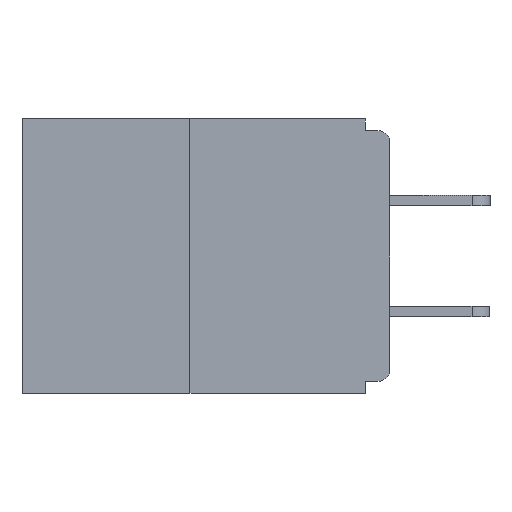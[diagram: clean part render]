
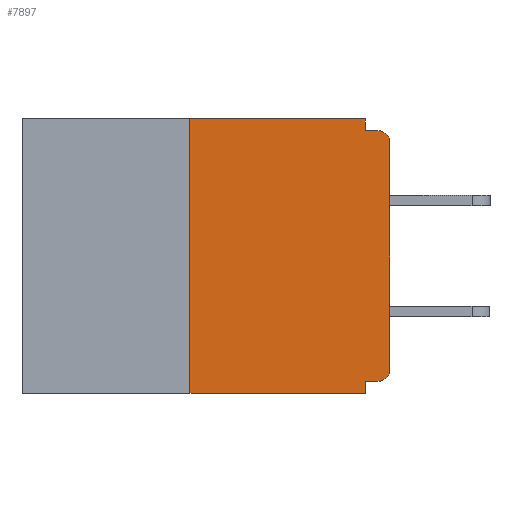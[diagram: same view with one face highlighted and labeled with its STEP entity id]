
A CAD part, left-side view. The second image highlights one B-rep face of the part: STEP entity #7897.
In plain terms, the highlighted planar face has unit normal (-1, 0, 0).
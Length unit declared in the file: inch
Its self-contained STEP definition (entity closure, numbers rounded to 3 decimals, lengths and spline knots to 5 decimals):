
#961 = AXIS2_PLACEMENT_3D ( 'NONE', #22468, #20516, #13202 ) ;
#1058 = CARTESIAN_POINT ( 'NONE',  ( 0., 0.015, -0.313 ) ) ;
#1637 = DIRECTION ( 'NONE',  ( 0., 0., -1. ) ) ;
#2032 = DIRECTION ( 'NONE',  ( 0., 0., 1. ) ) ;
#2103 = CARTESIAN_POINT ( 'NONE',  ( 0., 0.46, 0. ) ) ;
#2160 = VECTOR ( 'NONE', #12771, 39.37008 ) ;
#2252 = CARTESIAN_POINT ( 'NONE',  ( 0., 0.031, -0.015 ) ) ;
#2762 = CARTESIAN_POINT ( 'NONE',  ( 0., 0., -0.328 ) ) ;
#2796 = VERTEX_POINT ( 'NONE', #6605 ) ;
#4033 = CARTESIAN_POINT ( 'NONE',  ( 0., 0., -0.313 ) ) ;
#4126 = LINE ( 'NONE', #11154, #8659 ) ;
#4278 = VECTOR ( 'NONE', #19106, 39.37008 ) ;
#4566 = CARTESIAN_POINT ( 'NONE',  ( 0., 0.015, -0.328 ) ) ;
#4717 = CARTESIAN_POINT ( 'NONE',  ( 0., 0.46, 0. ) ) ;
#4772 = CARTESIAN_POINT ( 'NONE',  ( 0., 0.031, -0.328 ) ) ;
#4995 = LINE ( 'NONE', #21578, #2160 ) ;
#5096 = CARTESIAN_POINT ( 'NONE',  ( 0., 0.031, -0.343 ) ) ;
#5404 = LINE ( 'NONE', #2762, #10468 ) ;
#5552 = CARTESIAN_POINT ( 'NONE',  ( 0., 0.25, 0. ) ) ;
#5697 = DIRECTION ( 'NONE',  ( 0., 0., -1. ) ) ;
#5854 = PLANE ( 'NONE',  #20369 ) ;
#5968 = LINE ( 'NONE', #4717, #4278 ) ;
#6163 = DIRECTION ( 'NONE',  ( 0., 0., -1. ) ) ;
#6268 = CIRCLE ( 'NONE', #8490, 0.015 ) ;
#6605 = CARTESIAN_POINT ( 'NONE',  ( 0., 0.25, 0. ) ) ;
#6688 = ORIENTED_EDGE ( 'NONE', *, *, #12822, .F. ) ;
#6816 = VERTEX_POINT ( 'NONE', #20747 ) ;
#7607 = VECTOR ( 'NONE', #19515, 39.37008 ) ;
#7686 = EDGE_CURVE ( 'NONE', #12947, #17990, #20958, .T. ) ;
#7765 = VECTOR ( 'NONE', #9118, 39.37008 ) ;
#7801 = VERTEX_POINT ( 'NONE', #2252 ) ;
#7897 = ADVANCED_FACE ( 'NONE', ( #8918 ), #5854, .F. ) ;
#7995 = LINE ( 'NONE', #5096, #11646 ) ;
#8466 = ORIENTED_EDGE ( 'NONE', *, *, #16003, .T. ) ;
#8490 = AXIS2_PLACEMENT_3D ( 'NONE', #1058, #17100, #6163 ) ;
#8659 = VECTOR ( 'NONE', #18235, 39.37008 ) ;
#8673 = VECTOR ( 'NONE', #2032, 39.37008 ) ;
#8918 = FACE_OUTER_BOUND ( 'NONE', #12753, .T. ) ;
#8960 = CARTESIAN_POINT ( 'NONE',  ( 0., 0.46, -0.343 ) ) ;
#9011 = EDGE_CURVE ( 'NONE', #11687, #12338, #15322, .T. ) ;
#9102 = VERTEX_POINT ( 'NONE', #4566 ) ;
#9118 = DIRECTION ( 'NONE',  ( 0., -1., 0. ) ) ;
#9491 = LINE ( 'NONE', #5552, #8673 ) ;
#9560 = LINE ( 'NONE', #19280, #7607 ) ;
#9911 = CARTESIAN_POINT ( 'NONE',  ( 0., 0.031, -0.343 ) ) ;
#9999 = DIRECTION ( 'NONE',  ( 0., 1., 0. ) ) ;
#10468 = VECTOR ( 'NONE', #9999, 39.37008 ) ;
#11154 = CARTESIAN_POINT ( 'NONE',  ( 0., 0., 0. ) ) ;
#11646 = VECTOR ( 'NONE', #1637, 39.37008 ) ;
#11687 = VERTEX_POINT ( 'NONE', #15221 ) ;
#12338 = VERTEX_POINT ( 'NONE', #18419 ) ;
#12550 = VERTEX_POINT ( 'NONE', #4772 ) ;
#12753 = EDGE_LOOP ( 'NONE', ( #18655, #6688, #15230, #17712, #17539, #8466, #20015, #14508, #19276, #15536 ) ) ;
#12771 = DIRECTION ( 'NONE',  ( 0., 0., -1. ) ) ;
#12822 = EDGE_CURVE ( 'NONE', #12947, #2796, #9491, .T. ) ;
#12947 = VERTEX_POINT ( 'NONE', #20391 ) ;
#13202 = DIRECTION ( 'NONE',  ( 0., 0., -1. ) ) ;
#14508 = ORIENTED_EDGE ( 'NONE', *, *, #9011, .T. ) ;
#14705 = DIRECTION ( 'NONE',  ( 1., 0., 0. ) ) ;
#15221 = CARTESIAN_POINT ( 'NONE',  ( 0., 0., -0.03 ) ) ;
#15230 = ORIENTED_EDGE ( 'NONE', *, *, #7686, .T. ) ;
#15322 = CIRCLE ( 'NONE', #961, 0.015 ) ;
#15536 = ORIENTED_EDGE ( 'NONE', *, *, #17515, .F. ) ;
#16003 = EDGE_CURVE ( 'NONE', #9102, #20928, #6268, .T. ) ;
#16598 = EDGE_CURVE ( 'NONE', #9102, #12550, #5404, .T. ) ;
#16624 = EDGE_CURVE ( 'NONE', #2796, #6816, #5968, .T. ) ;
#17100 = DIRECTION ( 'NONE',  ( -1., 0., 0. ) ) ;
#17515 = EDGE_CURVE ( 'NONE', #6816, #7801, #4995, .T. ) ;
#17539 = ORIENTED_EDGE ( 'NONE', *, *, #16598, .F. ) ;
#17712 = ORIENTED_EDGE ( 'NONE', *, *, #19796, .F. ) ;
#17990 = VERTEX_POINT ( 'NONE', #9911 ) ;
#18195 = EDGE_CURVE ( 'NONE', #20928, #11687, #4126, .T. ) ;
#18235 = DIRECTION ( 'NONE',  ( 0., 0., 1. ) ) ;
#18419 = CARTESIAN_POINT ( 'NONE',  ( 0., 0.015, -0.015 ) ) ;
#18655 = ORIENTED_EDGE ( 'NONE', *, *, #16624, .F. ) ;
#19106 = DIRECTION ( 'NONE',  ( 0., -1., 0. ) ) ;
#19276 = ORIENTED_EDGE ( 'NONE', *, *, #22598, .F. ) ;
#19280 = CARTESIAN_POINT ( 'NONE',  ( 0., 0., -0.015 ) ) ;
#19515 = DIRECTION ( 'NONE',  ( 0., -1., 0. ) ) ;
#19796 = EDGE_CURVE ( 'NONE', #12550, #17990, #7995, .T. ) ;
#20015 = ORIENTED_EDGE ( 'NONE', *, *, #18195, .T. ) ;
#20369 = AXIS2_PLACEMENT_3D ( 'NONE', #2103, #14705, #5697 ) ;
#20391 = CARTESIAN_POINT ( 'NONE',  ( 0., 0.25, -0.343 ) ) ;
#20516 = DIRECTION ( 'NONE',  ( -1., 0., 0. ) ) ;
#20747 = CARTESIAN_POINT ( 'NONE',  ( 0., 0.031, 0. ) ) ;
#20928 = VERTEX_POINT ( 'NONE', #4033 ) ;
#20958 = LINE ( 'NONE', #8960, #7765 ) ;
#21578 = CARTESIAN_POINT ( 'NONE',  ( 0., 0.031, 0. ) ) ;
#22468 = CARTESIAN_POINT ( 'NONE',  ( 0., 0.015, -0.03 ) ) ;
#22598 = EDGE_CURVE ( 'NONE', #7801, #12338, #9560, .T. ) ;
